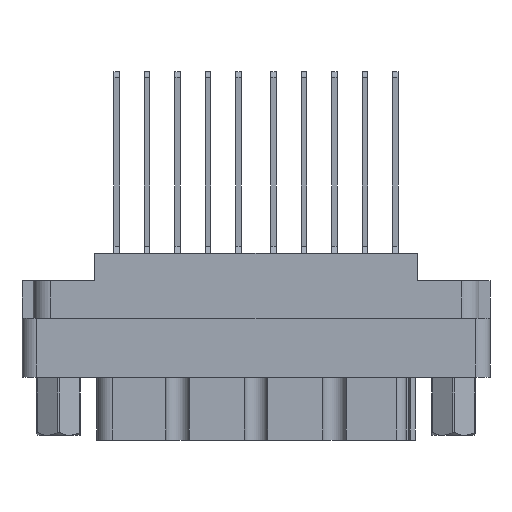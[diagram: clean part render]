
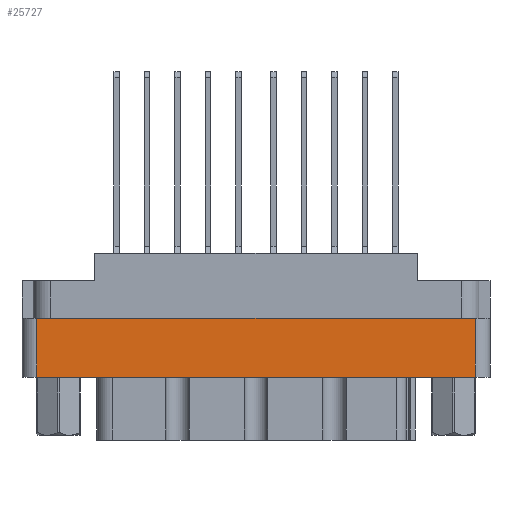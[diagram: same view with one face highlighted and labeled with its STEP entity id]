
A CAD part, front view. The second image highlights one B-rep face of the part: STEP entity #25727.
In plain terms, the highlighted planar face has unit normal (0, -1, 0).
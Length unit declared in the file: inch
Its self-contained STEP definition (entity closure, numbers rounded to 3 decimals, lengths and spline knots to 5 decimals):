
#1778 = VECTOR ( 'NONE', #42288, 39.37008 ) ;
#2121 = DIRECTION ( 'NONE',  ( 0., -1., 0. ) ) ;
#4457 = DIRECTION ( 'NONE',  ( 0., 0., -1. ) ) ;
#7484 = VERTEX_POINT ( 'NONE', #24369 ) ;
#8033 = CARTESIAN_POINT ( 'NONE',  ( -0.938, -0.438, -0.277 ) ) ;
#9200 = LINE ( 'NONE', #12272, #47098 ) ;
#11166 = LINE ( 'NONE', #41709, #44459 ) ;
#12217 = EDGE_CURVE ( 'NONE', #36719, #7484, #32840, .T. ) ;
#12272 = CARTESIAN_POINT ( 'NONE',  ( 0., -0.438, -0.277 ) ) ;
#12926 = CARTESIAN_POINT ( 'NONE',  ( 0.938, -0.438, -0.798 ) ) ;
#13090 = CARTESIAN_POINT ( 'NONE',  ( 0., -0.438, -0.529 ) ) ;
#15878 = VERTEX_POINT ( 'NONE', #8033 ) ;
#17210 = DIRECTION ( 'NONE',  ( 0., 0., -1. ) ) ;
#17905 = VECTOR ( 'NONE', #24938, 39.37008 ) ;
#18023 = ORIENTED_EDGE ( 'NONE', *, *, #12217, .T. ) ;
#18231 = EDGE_LOOP ( 'NONE', ( #46168, #28278, #24084, #18023 ) ) ;
#20694 = FACE_OUTER_BOUND ( 'NONE', #18231, .T. ) ;
#23105 = AXIS2_PLACEMENT_3D ( 'NONE', #31519, #2121, #17210 ) ;
#24084 = ORIENTED_EDGE ( 'NONE', *, *, #31520, .F. ) ;
#24256 = PLANE ( 'NONE',  #23105 ) ;
#24369 = CARTESIAN_POINT ( 'NONE',  ( 0.938, -0.438, -0.277 ) ) ;
#24938 = DIRECTION ( 'NONE',  ( 0., 0., 1. ) ) ;
#25727 = ADVANCED_FACE ( 'NONE', ( #20694 ), #24256, .T. ) ;
#27068 = LINE ( 'NONE', #13090, #1778 ) ;
#27328 = CARTESIAN_POINT ( 'NONE',  ( 0.938, -0.438, -0.529 ) ) ;
#28278 = ORIENTED_EDGE ( 'NONE', *, *, #43618, .T. ) ;
#31491 = EDGE_CURVE ( 'NONE', #15878, #7484, #9200, .T. ) ;
#31519 = CARTESIAN_POINT ( 'NONE',  ( -1., -0.438, -0.798 ) ) ;
#31520 = EDGE_CURVE ( 'NONE', #36719, #46112, #27068, .T. ) ;
#32840 = LINE ( 'NONE', #12926, #17905 ) ;
#34760 = DIRECTION ( 'NONE',  ( 1., 0., 0. ) ) ;
#36719 = VERTEX_POINT ( 'NONE', #27328 ) ;
#40065 = CARTESIAN_POINT ( 'NONE',  ( -0.938, -0.438, -0.529 ) ) ;
#41709 = CARTESIAN_POINT ( 'NONE',  ( -0.938, -0.438, -0.798 ) ) ;
#42288 = DIRECTION ( 'NONE',  ( -1., 0., 0. ) ) ;
#43618 = EDGE_CURVE ( 'NONE', #15878, #46112, #11166, .T. ) ;
#44459 = VECTOR ( 'NONE', #4457, 39.37008 ) ;
#46112 = VERTEX_POINT ( 'NONE', #40065 ) ;
#46168 = ORIENTED_EDGE ( 'NONE', *, *, #31491, .F. ) ;
#47098 = VECTOR ( 'NONE', #34760, 39.37008 ) ;
